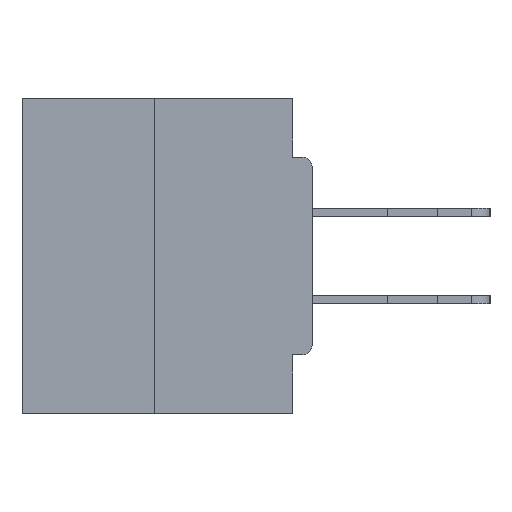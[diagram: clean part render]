
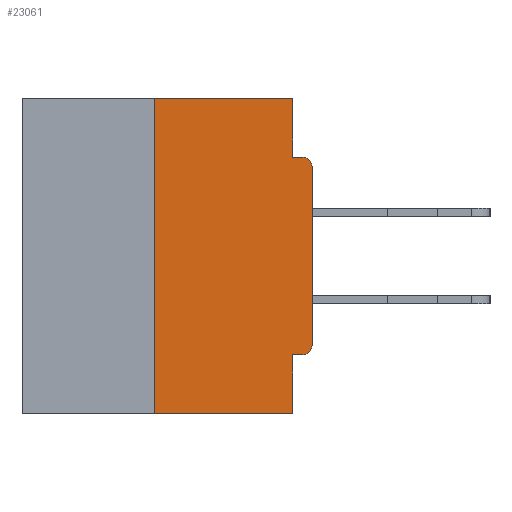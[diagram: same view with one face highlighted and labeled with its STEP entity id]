
A CAD part, left-side view. The second image highlights one B-rep face of the part: STEP entity #23061.
In plain terms, the highlighted planar face has unit normal (-1, 0, 0).
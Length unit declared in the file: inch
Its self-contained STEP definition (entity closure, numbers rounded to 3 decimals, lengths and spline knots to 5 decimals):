
#1170 = AXIS2_PLACEMENT_3D ( 'NONE', #23721, #1490, #7102 ) ;
#1442 = EDGE_CURVE ( 'NONE', #20665, #18108, #17009, .T. ) ;
#1490 = DIRECTION ( 'NONE',  ( 1., 0., 0. ) ) ;
#1652 = CARTESIAN_POINT ( 'NONE',  ( 0., 0.031, -0.0935 ) ) ;
#1846 = CARTESIAN_POINT ( 'NONE',  ( 0., 0.031, -0.4065 ) ) ;
#2238 = ORIENTED_EDGE ( 'NONE', *, *, #31289, .T. ) ;
#3364 = ORIENTED_EDGE ( 'NONE', *, *, #33702, .F. ) ;
#3403 = CARTESIAN_POINT ( 'NONE',  ( 0., 0.031, 0. ) ) ;
#3809 = DIRECTION ( 'NONE',  ( 0., -1., 0. ) ) ;
#3837 = VERTEX_POINT ( 'NONE', #1846 ) ;
#4299 = CARTESIAN_POINT ( 'NONE',  ( 0., 0.015, -0.4065 ) ) ;
#4628 = DIRECTION ( 'NONE',  ( 0., -1., 0. ) ) ;
#4922 = EDGE_CURVE ( 'NONE', #6186, #15690, #34767, .T. ) ;
#6186 = VERTEX_POINT ( 'NONE', #4299 ) ;
#6424 = LINE ( 'NONE', #21127, #27242 ) ;
#6559 = CIRCLE ( 'NONE', #12275, 0.015 ) ;
#7012 = EDGE_CURVE ( 'NONE', #6186, #3837, #34158, .T. ) ;
#7102 = DIRECTION ( 'NONE',  ( 0., 0., -1. ) ) ;
#8920 = EDGE_CURVE ( 'NONE', #18108, #28531, #30536, .T. ) ;
#9015 = CARTESIAN_POINT ( 'NONE',  ( 0., 0.25, -0.5 ) ) ;
#9312 = VECTOR ( 'NONE', #33015, 39.37008 ) ;
#10969 = CARTESIAN_POINT ( 'NONE',  ( 0., 0., -0.1085 ) ) ;
#11626 = EDGE_CURVE ( 'NONE', #31730, #20665, #12427, .T. ) ;
#12275 = AXIS2_PLACEMENT_3D ( 'NONE', #28977, #23572, #26597 ) ;
#12427 = LINE ( 'NONE', #23516, #33693 ) ;
#13009 = VERTEX_POINT ( 'NONE', #16132 ) ;
#13508 = VECTOR ( 'NONE', #20670, 39.37008 ) ;
#13555 = DIRECTION ( 'NONE',  ( 0., -1., 0. ) ) ;
#13878 = ORIENTED_EDGE ( 'NONE', *, *, #7012, .F. ) ;
#14149 = ORIENTED_EDGE ( 'NONE', *, *, #8920, .F. ) ;
#14442 = AXIS2_PLACEMENT_3D ( 'NONE', #23377, #23136, #28781 ) ;
#15163 = VECTOR ( 'NONE', #13555, 39.37008 ) ;
#15378 = DIRECTION ( 'NONE',  ( 0., 0., -1. ) ) ;
#15690 = VERTEX_POINT ( 'NONE', #17474 ) ;
#16128 = VERTEX_POINT ( 'NONE', #10969 ) ;
#16132 = CARTESIAN_POINT ( 'NONE',  ( 0., 0.015, -0.0935 ) ) ;
#16414 = ORIENTED_EDGE ( 'NONE', *, *, #31991, .T. ) ;
#17009 = LINE ( 'NONE', #26267, #31733 ) ;
#17474 = CARTESIAN_POINT ( 'NONE',  ( 0., 0., -0.3915 ) ) ;
#18108 = VERTEX_POINT ( 'NONE', #3403 ) ;
#18201 = VECTOR ( 'NONE', #4628, 39.37008 ) ;
#18409 = ORIENTED_EDGE ( 'NONE', *, *, #11626, .F. ) ;
#19516 = LINE ( 'NONE', #21171, #18201 ) ;
#20562 = PLANE ( 'NONE',  #1170 ) ;
#20665 = VERTEX_POINT ( 'NONE', #28294 ) ;
#20670 = DIRECTION ( 'NONE',  ( 0., 0., 1. ) ) ;
#21127 = CARTESIAN_POINT ( 'NONE',  ( 0., 0.031, -0.5 ) ) ;
#21171 = CARTESIAN_POINT ( 'NONE',  ( 0., 0., -0.0935 ) ) ;
#23061 = ADVANCED_FACE ( 'NONE', ( #35823 ), #20562, .F. ) ;
#23136 = DIRECTION ( 'NONE',  ( -1., 0., 0. ) ) ;
#23377 = CARTESIAN_POINT ( 'NONE',  ( 0., 0.015, -0.3915 ) ) ;
#23516 = CARTESIAN_POINT ( 'NONE',  ( 0., 0.25, 0. ) ) ;
#23572 = DIRECTION ( 'NONE',  ( -1., 0., 0. ) ) ;
#23701 = CARTESIAN_POINT ( 'NONE',  ( 0., 0., 0. ) ) ;
#23721 = CARTESIAN_POINT ( 'NONE',  ( 0., 0.46, 0. ) ) ;
#24332 = LINE ( 'NONE', #32464, #15163 ) ;
#25543 = ORIENTED_EDGE ( 'NONE', *, *, #4922, .T. ) ;
#26040 = ORIENTED_EDGE ( 'NONE', *, *, #1442, .F. ) ;
#26267 = CARTESIAN_POINT ( 'NONE',  ( 0., 0.46, 0. ) ) ;
#26597 = DIRECTION ( 'NONE',  ( 0., 0., -1. ) ) ;
#26905 = CARTESIAN_POINT ( 'NONE',  ( 0., 0.031, -0.5 ) ) ;
#27037 = ORIENTED_EDGE ( 'NONE', *, *, #31189, .T. ) ;
#27242 = VECTOR ( 'NONE', #15378, 39.37008 ) ;
#28294 = CARTESIAN_POINT ( 'NONE',  ( 0., 0.25, 0. ) ) ;
#28509 = ORIENTED_EDGE ( 'NONE', *, *, #33168, .F. ) ;
#28531 = VERTEX_POINT ( 'NONE', #1652 ) ;
#28560 = CARTESIAN_POINT ( 'NONE',  ( 0., 0., -0.4065 ) ) ;
#28781 = DIRECTION ( 'NONE',  ( 0., 0., -1. ) ) ;
#28799 = DIRECTION ( 'NONE',  ( 0., 1., 0. ) ) ;
#28977 = CARTESIAN_POINT ( 'NONE',  ( 0., 0.015, -0.1085 ) ) ;
#29295 = DIRECTION ( 'NONE',  ( 0., 0., 1. ) ) ;
#30536 = LINE ( 'NONE', #35410, #9312 ) ;
#31189 = EDGE_CURVE ( 'NONE', #15690, #16128, #32152, .T. ) ;
#31289 = EDGE_CURVE ( 'NONE', #16128, #13009, #6559, .T. ) ;
#31730 = VERTEX_POINT ( 'NONE', #9015 ) ;
#31733 = VECTOR ( 'NONE', #3809, 39.37008 ) ;
#31991 = EDGE_CURVE ( 'NONE', #31730, #34280, #24332, .T. ) ;
#32152 = LINE ( 'NONE', #23701, #13508 ) ;
#32464 = CARTESIAN_POINT ( 'NONE',  ( 0., 0.46, -0.5 ) ) ;
#32495 = EDGE_LOOP ( 'NONE', ( #26040, #18409, #16414, #3364, #13878, #25543, #27037, #2238, #28509, #14149 ) ) ;
#32904 = VECTOR ( 'NONE', #28799, 39.37008 ) ;
#33015 = DIRECTION ( 'NONE',  ( 0., 0., -1. ) ) ;
#33168 = EDGE_CURVE ( 'NONE', #28531, #13009, #19516, .T. ) ;
#33693 = VECTOR ( 'NONE', #29295, 39.37008 ) ;
#33702 = EDGE_CURVE ( 'NONE', #3837, #34280, #6424, .T. ) ;
#34158 = LINE ( 'NONE', #28560, #32904 ) ;
#34280 = VERTEX_POINT ( 'NONE', #26905 ) ;
#34767 = CIRCLE ( 'NONE', #14442, 0.015 ) ;
#35410 = CARTESIAN_POINT ( 'NONE',  ( 0., 0.031, 0. ) ) ;
#35823 = FACE_OUTER_BOUND ( 'NONE', #32495, .T. ) ;
